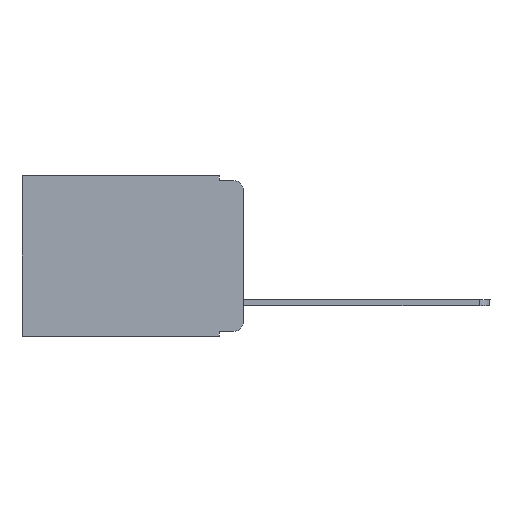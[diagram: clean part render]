
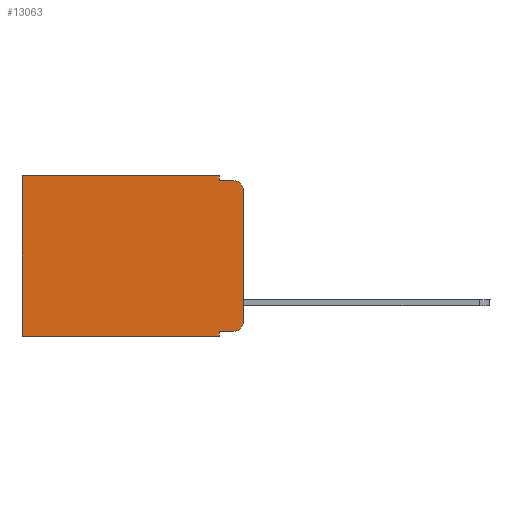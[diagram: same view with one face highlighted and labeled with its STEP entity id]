
A CAD part, left-side view. The second image highlights one B-rep face of the part: STEP entity #13063.
In plain terms, the highlighted planar face has unit normal (-1, 0, 0).
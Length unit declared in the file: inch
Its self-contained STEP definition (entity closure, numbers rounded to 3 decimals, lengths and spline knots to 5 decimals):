
#65 = CARTESIAN_POINT ( 'NONE',  ( 0.298, 0.02, -0.313 ) ) ;
#319 = VECTOR ( 'NONE', #1435, 39.37008 ) ;
#671 = CARTESIAN_POINT ( 'NONE',  ( 0.298, 0.02, -0.333 ) ) ;
#882 = VECTOR ( 'NONE', #14062, 39.37008 ) ;
#909 = EDGE_CURVE ( 'NONE', #19295, #9362, #12792, .T. ) ;
#1229 = ORIENTED_EDGE ( 'NONE', *, *, #8356, .F. ) ;
#1317 = DIRECTION ( 'NONE',  ( 0., 0., -1. ) ) ;
#1435 = DIRECTION ( 'NONE',  ( 0., 0., -1. ) ) ;
#1483 = PLANE ( 'NONE',  #6736 ) ;
#1655 = DIRECTION ( 'NONE',  ( -1., 0., 0. ) ) ;
#1959 = LINE ( 'NONE', #7619, #2452 ) ;
#2192 = DIRECTION ( 'NONE',  ( 0., 1., 0. ) ) ;
#2452 = VECTOR ( 'NONE', #14031, 39.37008 ) ;
#3130 = CARTESIAN_POINT ( 'NONE',  ( 0.298, 0.473, 0. ) ) ;
#3186 = EDGE_CURVE ( 'NONE', #16669, #3498, #15553, .T. ) ;
#3498 = VERTEX_POINT ( 'NONE', #11867 ) ;
#3622 = VERTEX_POINT ( 'NONE', #12266 ) ;
#4054 = EDGE_CURVE ( 'NONE', #3622, #3498, #18078, .T. ) ;
#4434 = EDGE_CURVE ( 'NONE', #10896, #16669, #6183, .T. ) ;
#4443 = EDGE_LOOP ( 'NONE', ( #5148, #11440, #6032, #14223, #15630, #5433, #17687, #1229, #5268, #6270 ) ) ;
#4928 = EDGE_CURVE ( 'NONE', #13527, #15704, #17476, .T. ) ;
#5148 = ORIENTED_EDGE ( 'NONE', *, *, #10948, .F. ) ;
#5268 = ORIENTED_EDGE ( 'NONE', *, *, #6074, .T. ) ;
#5433 = ORIENTED_EDGE ( 'NONE', *, *, #4928, .T. ) ;
#5438 = CARTESIAN_POINT ( 'NONE',  ( 0.298, 0., -0.313 ) ) ;
#5522 = CARTESIAN_POINT ( 'NONE',  ( 0.298, 0., 0. ) ) ;
#5804 = DIRECTION ( 'NONE',  ( 0., 0., -1. ) ) ;
#6032 = ORIENTED_EDGE ( 'NONE', *, *, #3186, .F. ) ;
#6038 = DIRECTION ( 'NONE',  ( 0., 0., -1. ) ) ;
#6074 = EDGE_CURVE ( 'NONE', #11114, #19295, #1959, .T. ) ;
#6183 = LINE ( 'NONE', #13401, #319 ) ;
#6270 = ORIENTED_EDGE ( 'NONE', *, *, #909, .T. ) ;
#6286 = CARTESIAN_POINT ( 'NONE',  ( 0.298, 0.051, -0.01 ) ) ;
#6613 = DIRECTION ( 'NONE',  ( 0., 0., -1. ) ) ;
#6705 = VERTEX_POINT ( 'NONE', #8850 ) ;
#6736 = AXIS2_PLACEMENT_3D ( 'NONE', #10288, #13558, #6038 ) ;
#7260 = LINE ( 'NONE', #17637, #10100 ) ;
#7460 = VECTOR ( 'NONE', #13268, 39.37008 ) ;
#7597 = DIRECTION ( 'NONE',  ( -1., 0., 0. ) ) ;
#7619 = CARTESIAN_POINT ( 'NONE',  ( 0.298, 0.051, -0.333 ) ) ;
#8356 = EDGE_CURVE ( 'NONE', #11114, #6705, #7260, .T. ) ;
#8850 = CARTESIAN_POINT ( 'NONE',  ( 0.298, 0.051, -0.343 ) ) ;
#8977 = CARTESIAN_POINT ( 'NONE',  ( 0.298, 0.051, -0.333 ) ) ;
#9362 = VERTEX_POINT ( 'NONE', #5438 ) ;
#9537 = VECTOR ( 'NONE', #13230, 39.37008 ) ;
#9948 = VECTOR ( 'NONE', #6613, 39.37008 ) ;
#10100 = VECTOR ( 'NONE', #1317, 39.37008 ) ;
#10288 = CARTESIAN_POINT ( 'NONE',  ( 0.298, 0., 0. ) ) ;
#10847 = CARTESIAN_POINT ( 'NONE',  ( 0.298, 0.02, -0.03 ) ) ;
#10896 = VERTEX_POINT ( 'NONE', #14035 ) ;
#10948 = EDGE_CURVE ( 'NONE', #3622, #9362, #19350, .T. ) ;
#11114 = VERTEX_POINT ( 'NONE', #8977 ) ;
#11440 = ORIENTED_EDGE ( 'NONE', *, *, #4054, .T. ) ;
#11867 = CARTESIAN_POINT ( 'NONE',  ( 0.298, 0.02, -0.01 ) ) ;
#12266 = CARTESIAN_POINT ( 'NONE',  ( 0.298, 0., -0.03 ) ) ;
#12683 = LINE ( 'NONE', #15751, #14066 ) ;
#12792 = CIRCLE ( 'NONE', #13100, 0.02 ) ;
#13063 = ADVANCED_FACE ( 'NONE', ( #19283 ), #1483, .F. ) ;
#13100 = AXIS2_PLACEMENT_3D ( 'NONE', #65, #7597, #5804 ) ;
#13230 = DIRECTION ( 'NONE',  ( 0., 0., -1. ) ) ;
#13268 = DIRECTION ( 'NONE',  ( 0., 1., 0. ) ) ;
#13401 = CARTESIAN_POINT ( 'NONE',  ( 0.298, 0.051, 0. ) ) ;
#13527 = VERTEX_POINT ( 'NONE', #3130 ) ;
#13558 = DIRECTION ( 'NONE',  ( 1., 0., 0. ) ) ;
#13830 = DIRECTION ( 'NONE',  ( 0., 0., -1. ) ) ;
#14031 = DIRECTION ( 'NONE',  ( 0., -1., 0. ) ) ;
#14035 = CARTESIAN_POINT ( 'NONE',  ( 0.298, 0.051, 0. ) ) ;
#14062 = DIRECTION ( 'NONE',  ( 0., -1., 0. ) ) ;
#14066 = VECTOR ( 'NONE', #2192, 39.37008 ) ;
#14223 = ORIENTED_EDGE ( 'NONE', *, *, #4434, .F. ) ;
#14567 = CARTESIAN_POINT ( 'NONE',  ( 0.298, 0., 0. ) ) ;
#15553 = LINE ( 'NONE', #16927, #882 ) ;
#15630 = ORIENTED_EDGE ( 'NONE', *, *, #17416, .T. ) ;
#15704 = VERTEX_POINT ( 'NONE', #18406 ) ;
#15751 = CARTESIAN_POINT ( 'NONE',  ( 0.298, 0., -0.343 ) ) ;
#16669 = VERTEX_POINT ( 'NONE', #6286 ) ;
#16927 = CARTESIAN_POINT ( 'NONE',  ( 0.298, 0.051, -0.01 ) ) ;
#17272 = EDGE_CURVE ( 'NONE', #6705, #15704, #12683, .T. ) ;
#17416 = EDGE_CURVE ( 'NONE', #10896, #13527, #19008, .T. ) ;
#17476 = LINE ( 'NONE', #18753, #9948 ) ;
#17637 = CARTESIAN_POINT ( 'NONE',  ( 0.298, 0.051, 0. ) ) ;
#17687 = ORIENTED_EDGE ( 'NONE', *, *, #17272, .F. ) ;
#18078 = CIRCLE ( 'NONE', #18383, 0.02 ) ;
#18383 = AXIS2_PLACEMENT_3D ( 'NONE', #10847, #1655, #13830 ) ;
#18406 = CARTESIAN_POINT ( 'NONE',  ( 0.298, 0.473, -0.343 ) ) ;
#18753 = CARTESIAN_POINT ( 'NONE',  ( 0.298, 0.473, 0. ) ) ;
#19008 = LINE ( 'NONE', #14567, #7460 ) ;
#19283 = FACE_OUTER_BOUND ( 'NONE', #4443, .T. ) ;
#19295 = VERTEX_POINT ( 'NONE', #671 ) ;
#19350 = LINE ( 'NONE', #5522, #9537 ) ;
